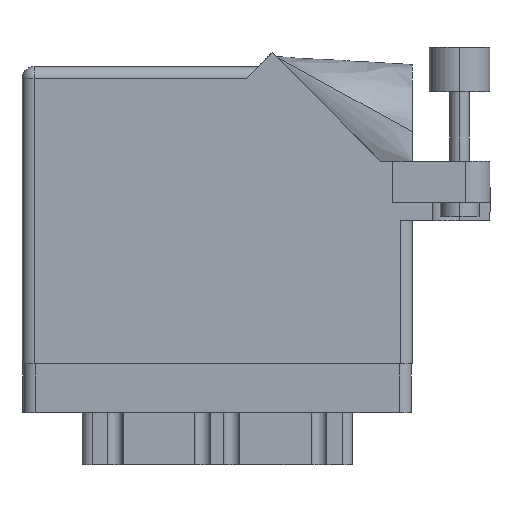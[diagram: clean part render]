
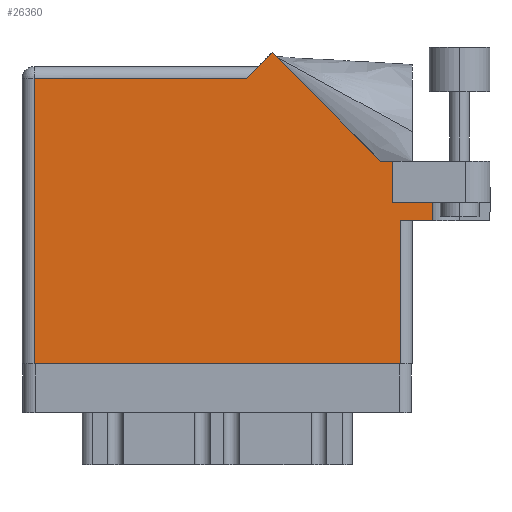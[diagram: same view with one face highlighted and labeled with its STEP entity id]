
A CAD part, front view. The second image highlights one B-rep face of the part: STEP entity #26360.
In plain terms, the highlighted face is planar.
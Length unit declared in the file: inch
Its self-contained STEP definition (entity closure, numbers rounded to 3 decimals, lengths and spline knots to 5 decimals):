
#212 = ORIENTED_EDGE ( 'NONE', *, *, #25027, .T. ) ;
#260 = LINE ( 'NONE', #14772, #1697 ) ;
#479 = VERTEX_POINT ( 'NONE', #23258 ) ;
#561 = ORIENTED_EDGE ( 'NONE', *, *, #20771, .T. ) ;
#1295 = DIRECTION ( 'NONE',  ( -0.707, 0.707, 0. ) ) ;
#1321 = DIRECTION ( 'NONE',  ( 1., 0., 0. ) ) ;
#1435 = DIRECTION ( 'NONE',  ( 0., 1., 0. ) ) ;
#1517 = VECTOR ( 'NONE', #7710, 39.37008 ) ;
#1697 = VECTOR ( 'NONE', #26130, 39.37008 ) ;
#2039 = DIRECTION ( 'NONE',  ( -1., 0., 0. ) ) ;
#2601 = ORIENTED_EDGE ( 'NONE', *, *, #3345, .F. ) ;
#3345 = EDGE_CURVE ( 'NONE', #22636, #11556, #4603, .T. ) ;
#3572 = ORIENTED_EDGE ( 'NONE', *, *, #9215, .T. ) ;
#3880 = DIRECTION ( 'NONE',  ( 1., 0., 0. ) ) ;
#4324 = ORIENTED_EDGE ( 'NONE', *, *, #14676, .F. ) ;
#4376 = CARTESIAN_POINT ( 'NONE',  ( 2.1115, 1.16177, 0. ) ) ;
#4603 = LINE ( 'NONE', #23685, #17357 ) ;
#5675 = EDGE_CURVE ( 'NONE', #479, #21273, #15876, .T. ) ;
#5898 = FACE_OUTER_BOUND ( 'NONE', #30157, .T. ) ;
#7162 = ORIENTED_EDGE ( 'NONE', *, *, #7733, .T. ) ;
#7232 = VECTOR ( 'NONE', #1295, 39.37008 ) ;
#7276 = LINE ( 'NONE', #28396, #23224 ) ;
#7445 = LINE ( 'NONE', #29355, #10919 ) ;
#7595 = VERTEX_POINT ( 'NONE', #31204 ) ;
#7710 = DIRECTION ( 'NONE',  ( 0., -1., 0. ) ) ;
#7733 = EDGE_CURVE ( 'NONE', #23441, #479, #12919, .T. ) ;
#7958 = CARTESIAN_POINT ( 'NONE',  ( 2.1115, 0.831, 0. ) ) ;
#8048 = CARTESIAN_POINT ( 'NONE',  ( 1.155, 1.468, 0. ) ) ;
#8723 = EDGE_CURVE ( 'NONE', #21315, #17676, #25430, .T. ) ;
#8883 = CARTESIAN_POINT ( 'NONE',  ( 0.062, 1.468, 0. ) ) ;
#9215 = EDGE_CURVE ( 'NONE', #26591, #23441, #260, .T. ) ;
#9325 = CARTESIAN_POINT ( 'NONE',  ( 1.84442, 1.044, 0. ) ) ;
#10032 = CARTESIAN_POINT ( 'NONE',  ( 1.28771, 1.60071, 0. ) ) ;
#10066 = CARTESIAN_POINT ( 'NONE',  ( 1.91, 1.044, 0. ) ) ;
#10086 = EDGE_CURVE ( 'NONE', #21273, #23398, #7445, .T. ) ;
#10318 = VECTOR ( 'NONE', #21097, 39.37008 ) ;
#10333 = ORIENTED_EDGE ( 'NONE', *, *, #18559, .T. ) ;
#10548 = CARTESIAN_POINT ( 'NONE',  ( 0.062, 0., 0. ) ) ;
#10919 = VECTOR ( 'NONE', #24781, 39.37008 ) ;
#11224 = VECTOR ( 'NONE', #1321, 39.37008 ) ;
#11556 = VERTEX_POINT ( 'NONE', #7958 ) ;
#11966 = ORIENTED_EDGE ( 'NONE', *, *, #10086, .T. ) ;
#12316 = ORIENTED_EDGE ( 'NONE', *, *, #8723, .T. ) ;
#12919 = LINE ( 'NONE', #10548, #1517 ) ;
#14229 = DIRECTION ( 'NONE',  ( 1., 0., 0. ) ) ;
#14676 = EDGE_CURVE ( 'NONE', #11556, #7595, #18422, .T. ) ;
#14772 = CARTESIAN_POINT ( 'NONE',  ( 0., 1.468, 0. ) ) ;
#15448 = AXIS2_PLACEMENT_3D ( 'NONE', #31060, #19713, #21615 ) ;
#15876 = LINE ( 'NONE', #25484, #22685 ) ;
#16104 = CARTESIAN_POINT ( 'NONE',  ( 1.91, 0.831, 0. ) ) ;
#17357 = VECTOR ( 'NONE', #14229, 39.37008 ) ;
#17676 = VERTEX_POINT ( 'NONE', #10032 ) ;
#17905 = LINE ( 'NONE', #29870, #11224 ) ;
#18422 = LINE ( 'NONE', #4376, #10318 ) ;
#18559 = EDGE_CURVE ( 'NONE', #27019, #21315, #26334, .T. ) ;
#19259 = DIRECTION ( 'NONE',  ( -0.707, -0.707, 0. ) ) ;
#19713 = DIRECTION ( 'NONE',  ( 0., 0., -1. ) ) ;
#20240 = PLANE ( 'NONE',  #15448 ) ;
#20771 = EDGE_CURVE ( 'NONE', #23398, #7595, #17905, .T. ) ;
#21097 = DIRECTION ( 'NONE',  ( 0., -1., 0. ) ) ;
#21273 = VERTEX_POINT ( 'NONE', #23200 ) ;
#21315 = VERTEX_POINT ( 'NONE', #9325 ) ;
#21615 = DIRECTION ( 'NONE',  ( -1., 0., 0. ) ) ;
#22602 = CARTESIAN_POINT ( 'NONE',  ( 1.84442, 1.044, 0. ) ) ;
#22636 = VERTEX_POINT ( 'NONE', #23937 ) ;
#22685 = VECTOR ( 'NONE', #3880, 39.37008 ) ;
#23200 = CARTESIAN_POINT ( 'NONE',  ( 1.948, 0., 0. ) ) ;
#23224 = VECTOR ( 'NONE', #19259, 39.37008 ) ;
#23258 = CARTESIAN_POINT ( 'NONE',  ( 0.062, 0., 0. ) ) ;
#23398 = VERTEX_POINT ( 'NONE', #25443 ) ;
#23441 = VERTEX_POINT ( 'NONE', #8883 ) ;
#23655 = CARTESIAN_POINT ( 'NONE',  ( 2.41, 1.044, 0. ) ) ;
#23685 = CARTESIAN_POINT ( 'NONE',  ( 1.91, 0.831, 0. ) ) ;
#23937 = CARTESIAN_POINT ( 'NONE',  ( 1.91, 0.831, 0. ) ) ;
#24781 = DIRECTION ( 'NONE',  ( 0., 1., 0. ) ) ;
#25027 = EDGE_CURVE ( 'NONE', #22636, #27019, #27943, .T. ) ;
#25052 = VECTOR ( 'NONE', #2039, 39.37008 ) ;
#25430 = LINE ( 'NONE', #22602, #7232 ) ;
#25443 = CARTESIAN_POINT ( 'NONE',  ( 1.948, 0.737, 0. ) ) ;
#25484 = CARTESIAN_POINT ( 'NONE',  ( 0., 0., 0. ) ) ;
#26130 = DIRECTION ( 'NONE',  ( -1., 0., 0. ) ) ;
#26334 = LINE ( 'NONE', #23655, #25052 ) ;
#26360 = ADVANCED_FACE ( 'NONE', ( #5898 ), #20240, .F. ) ;
#26591 = VERTEX_POINT ( 'NONE', #8048 ) ;
#27019 = VERTEX_POINT ( 'NONE', #10066 ) ;
#27943 = LINE ( 'NONE', #16104, #27958 ) ;
#27958 = VECTOR ( 'NONE', #1435, 39.37008 ) ;
#28396 = CARTESIAN_POINT ( 'NONE',  ( 1.217, 1.53, 0. ) ) ;
#29355 = CARTESIAN_POINT ( 'NONE',  ( 1.948, 0.737, 0. ) ) ;
#29382 = EDGE_CURVE ( 'NONE', #17676, #26591, #7276, .T. ) ;
#29870 = CARTESIAN_POINT ( 'NONE',  ( 2.01, 0.737, 0. ) ) ;
#30157 = EDGE_LOOP ( 'NONE', ( #31126, #11966, #561, #4324, #2601, #212, #10333, #12316, #30623, #3572, #7162 ) ) ;
#30623 = ORIENTED_EDGE ( 'NONE', *, *, #29382, .T. ) ;
#31060 = CARTESIAN_POINT ( 'NONE',  ( 0., 1.53, 0. ) ) ;
#31126 = ORIENTED_EDGE ( 'NONE', *, *, #5675, .T. ) ;
#31204 = CARTESIAN_POINT ( 'NONE',  ( 2.1115, 0.737, 0. ) ) ;
